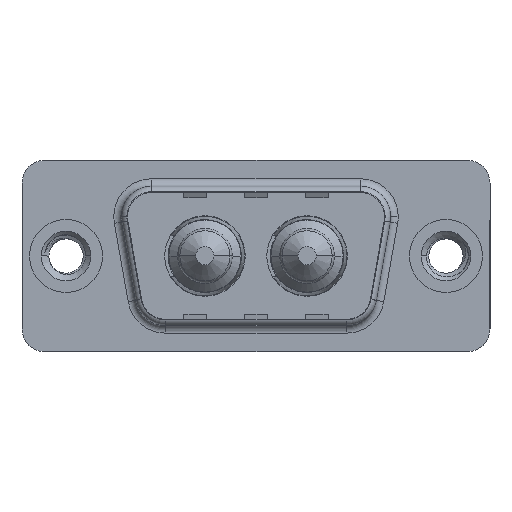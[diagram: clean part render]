
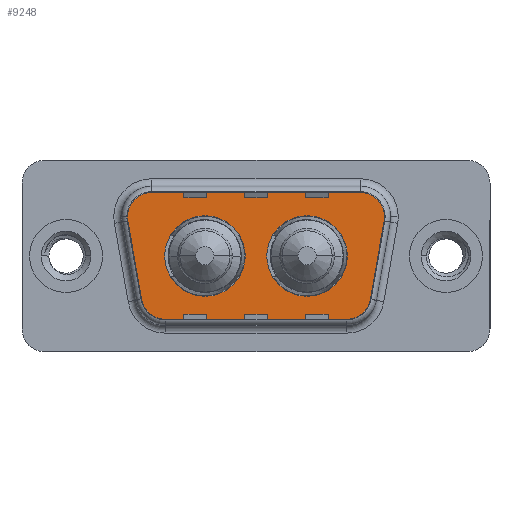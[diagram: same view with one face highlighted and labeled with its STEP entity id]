
A CAD part, top view. The second image highlights one B-rep face of the part: STEP entity #9248.
In plain terms, the highlighted planar face has unit normal (0, 0, 1).
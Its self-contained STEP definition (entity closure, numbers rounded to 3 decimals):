
#182 = CARTESIAN_POINT ( 'NONE',  ( 18.51, 0., 0. ) ) ;
#448 = DIRECTION ( 'NONE',  ( 1., 0., 0. ) ) ;
#459 = CARTESIAN_POINT ( 'NONE',  ( 3.466, 2.553, 0. ) ) ;
#536 = AXIS2_PLACEMENT_3D ( 'NONE', #2678, #3734, #14367 ) ;
#916 = VERTEX_POINT ( 'NONE', #13781 ) ;
#1003 = CARTESIAN_POINT ( 'NONE',  ( 4.489, -3.247, 0. ) ) ;
#1286 = LINE ( 'NONE', #11417, #12394 ) ;
#1322 = EDGE_CURVE ( 'NONE', #8747, #2855, #10840, .T. ) ;
#1399 = DIRECTION ( 'NONE',  ( 1., 0., 0. ) ) ;
#1548 = ORIENTED_EDGE ( 'NONE', *, *, #9249, .T. ) ;
#1556 = VERTEX_POINT ( 'NONE', #9598 ) ;
#1558 = CARTESIAN_POINT ( 'NONE',  ( 18.541, -4.9, 0. ) ) ;
#1772 = AXIS2_PLACEMENT_3D ( 'NONE', #13180, #13025, #5151 ) ;
#1902 = AXIS2_PLACEMENT_3D ( 'NONE', #4893, #12496, #5946 ) ;
#1916 = EDGE_CURVE ( 'NONE', #3289, #916, #9775, .T. ) ;
#2502 = AXIS2_PLACEMENT_3D ( 'NONE', #5964, #13618, #7005 ) ;
#2592 = ORIENTED_EDGE ( 'NONE', *, *, #5114, .T. ) ;
#2595 = CIRCLE ( 'NONE', #7024, 2. ) ;
#2678 = CARTESIAN_POINT ( 'NONE',  ( 19.564, 2.9, 0. ) ) ;
#2705 = AXIS2_PLACEMENT_3D ( 'NONE', #4806, #8030, #1399 ) ;
#2722 = DIRECTION ( 'NONE',  ( 0.174, -0.985, 0. ) ) ;
#2855 = VERTEX_POINT ( 'NONE', #13952 ) ;
#2955 = CARTESIAN_POINT ( 'NONE',  ( 21.534, 2.553, 0. ) ) ;
#3003 = ORIENTED_EDGE ( 'NONE', *, *, #4935, .T. ) ;
#3078 = VERTEX_POINT ( 'NONE', #5023 ) ;
#3113 = ORIENTED_EDGE ( 'NONE', *, *, #10744, .T. ) ;
#3155 = CARTESIAN_POINT ( 'NONE',  ( 5.436, 4.9, 0. ) ) ;
#3181 = DIRECTION ( 'NONE',  ( 1., 0., 0. ) ) ;
#3289 = VERTEX_POINT ( 'NONE', #182 ) ;
#3477 = ORIENTED_EDGE ( 'NONE', *, *, #8635, .F. ) ;
#3613 = AXIS2_PLACEMENT_3D ( 'NONE', #13808, #7171, #448 ) ;
#3653 = VERTEX_POINT ( 'NONE', #4293 ) ;
#3720 = CARTESIAN_POINT ( 'NONE',  ( 3.466, 2.553, 0. ) ) ;
#3734 = DIRECTION ( 'NONE',  ( 0., 0., 1. ) ) ;
#4022 = CARTESIAN_POINT ( 'NONE',  ( 20.511, -3.247, 0. ) ) ;
#4157 = CARTESIAN_POINT ( 'NONE',  ( 9.14, 0., 0. ) ) ;
#4293 = CARTESIAN_POINT ( 'NONE',  ( 19.564, 4.9, 0. ) ) ;
#4419 = FACE_OUTER_BOUND ( 'NONE', #11685, .T. ) ;
#4490 = AXIS2_PLACEMENT_3D ( 'NONE', #9485, #6674, #14259 ) ;
#4501 = CARTESIAN_POINT ( 'NONE',  ( 19.564, 2.9, 0. ) ) ;
#4584 = ORIENTED_EDGE ( 'NONE', *, *, #11109, .T. ) ;
#4750 = FACE_BOUND ( 'NONE', #14009, .T. ) ;
#4806 = CARTESIAN_POINT ( 'NONE',  ( 18.541, -2.9, 0. ) ) ;
#4855 = PLANE ( 'NONE',  #2705 ) ;
#4893 = CARTESIAN_POINT ( 'NONE',  ( 18.541, -2.9, 0. ) ) ;
#4935 = EDGE_CURVE ( 'NONE', #5301, #8747, #9007, .T. ) ;
#5023 = CARTESIAN_POINT ( 'NONE',  ( 11.79, 0., 0. ) ) ;
#5114 = EDGE_CURVE ( 'NONE', #6606, #8376, #10218, .T. ) ;
#5151 = DIRECTION ( 'NONE',  ( 1., 0., 0. ) ) ;
#5214 = DIRECTION ( 'NONE',  ( 0., 0., 1. ) ) ;
#5246 = DIRECTION ( 'NONE',  ( 1., 0., 0. ) ) ;
#5301 = VERTEX_POINT ( 'NONE', #4022 ) ;
#5488 = ORIENTED_EDGE ( 'NONE', *, *, #1322, .T. ) ;
#5946 = DIRECTION ( 'NONE',  ( 1., 0., 0. ) ) ;
#5964 = CARTESIAN_POINT ( 'NONE',  ( 9.14, 0., 0. ) ) ;
#6102 = ORIENTED_EDGE ( 'NONE', *, *, #6405, .T. ) ;
#6174 = EDGE_CURVE ( 'NONE', #8376, #1556, #8634, .T. ) ;
#6405 = EDGE_CURVE ( 'NONE', #2855, #3653, #2595, .T. ) ;
#6485 = CARTESIAN_POINT ( 'NONE',  ( 6.459, -4.9, 0. ) ) ;
#6562 = VERTEX_POINT ( 'NONE', #3155 ) ;
#6606 = VERTEX_POINT ( 'NONE', #459 ) ;
#6674 = DIRECTION ( 'NONE',  ( 0., 0., 1. ) ) ;
#6960 = CARTESIAN_POINT ( 'NONE',  ( 6.49, 0., 0. ) ) ;
#7005 = DIRECTION ( 'NONE',  ( 1., 0., 0. ) ) ;
#7024 = AXIS2_PLACEMENT_3D ( 'NONE', #4501, #14358, #13864 ) ;
#7074 = EDGE_LOOP ( 'NONE', ( #8391, #11410 ) ) ;
#7171 = DIRECTION ( 'NONE',  ( 0., 0., 1. ) ) ;
#7727 = ORIENTED_EDGE ( 'NONE', *, *, #12026, .F. ) ;
#8030 = DIRECTION ( 'NONE',  ( 0., 0., 1. ) ) ;
#8376 = VERTEX_POINT ( 'NONE', #1003 ) ;
#8391 = ORIENTED_EDGE ( 'NONE', *, *, #1916, .F. ) ;
#8438 = ORIENTED_EDGE ( 'NONE', *, *, #9271, .T. ) ;
#8634 = CIRCLE ( 'NONE', #4490, 2. ) ;
#8635 = EDGE_CURVE ( 'NONE', #10497, #3078, #12411, .T. ) ;
#8661 = VECTOR ( 'NONE', #9678, 1000. ) ;
#8747 = VERTEX_POINT ( 'NONE', #13722 ) ;
#8895 = AXIS2_PLACEMENT_3D ( 'NONE', #4157, #11777, #5246 ) ;
#9007 = LINE ( 'NONE', #2955, #8661 ) ;
#9226 = DIRECTION ( 'NONE',  ( -1., 0., 0. ) ) ;
#9248 = ADVANCED_FACE ( 'NONE', ( #10145, #4750, #4419 ), #4855, .T. ) ;
#9249 = EDGE_CURVE ( 'NONE', #11093, #5301, #9809, .T. ) ;
#9271 = EDGE_CURVE ( 'NONE', #3653, #6562, #1286, .T. ) ;
#9485 = CARTESIAN_POINT ( 'NONE',  ( 6.459, -2.9, 0. ) ) ;
#9504 = EDGE_CURVE ( 'NONE', #916, #3289, #11034, .T. ) ;
#9598 = CARTESIAN_POINT ( 'NONE',  ( 6.459, -4.9, 0. ) ) ;
#9678 = DIRECTION ( 'NONE',  ( 0.174, 0.985, 0. ) ) ;
#9775 = CIRCLE ( 'NONE', #1772, 2.65 ) ;
#9809 = CIRCLE ( 'NONE', #1902, 2. ) ;
#9962 = VECTOR ( 'NONE', #3181, 1000. ) ;
#10145 = FACE_BOUND ( 'NONE', #7074, .T. ) ;
#10218 = LINE ( 'NONE', #3720, #13482 ) ;
#10320 = LINE ( 'NONE', #6485, #9962 ) ;
#10497 = VERTEX_POINT ( 'NONE', #6960 ) ;
#10744 = EDGE_CURVE ( 'NONE', #1556, #11093, #10320, .T. ) ;
#10840 = CIRCLE ( 'NONE', #536, 2. ) ;
#11034 = CIRCLE ( 'NONE', #13023, 2.65 ) ;
#11093 = VERTEX_POINT ( 'NONE', #1558 ) ;
#11109 = EDGE_CURVE ( 'NONE', #6562, #6606, #13050, .T. ) ;
#11410 = ORIENTED_EDGE ( 'NONE', *, *, #9504, .F. ) ;
#11417 = CARTESIAN_POINT ( 'NONE',  ( 5.436, 4.9, 0. ) ) ;
#11685 = EDGE_LOOP ( 'NONE', ( #1548, #3003, #5488, #6102, #8438, #4584, #2592, #13427, #3113 ) ) ;
#11742 = CARTESIAN_POINT ( 'NONE',  ( 15.86, 0., 0. ) ) ;
#11777 = DIRECTION ( 'NONE',  ( 0., 0., 1. ) ) ;
#12026 = EDGE_CURVE ( 'NONE', #3078, #10497, #13035, .T. ) ;
#12394 = VECTOR ( 'NONE', #9226, 1000. ) ;
#12411 = CIRCLE ( 'NONE', #2502, 2.65 ) ;
#12496 = DIRECTION ( 'NONE',  ( 0., 0., 1. ) ) ;
#12813 = DIRECTION ( 'NONE',  ( 1., 0., 0. ) ) ;
#13023 = AXIS2_PLACEMENT_3D ( 'NONE', #11742, #5214, #12813 ) ;
#13025 = DIRECTION ( 'NONE',  ( 0., 0., 1. ) ) ;
#13035 = CIRCLE ( 'NONE', #8895, 2.65 ) ;
#13050 = CIRCLE ( 'NONE', #3613, 2. ) ;
#13180 = CARTESIAN_POINT ( 'NONE',  ( 15.86, 0., 0. ) ) ;
#13427 = ORIENTED_EDGE ( 'NONE', *, *, #6174, .T. ) ;
#13482 = VECTOR ( 'NONE', #2722, 1000. ) ;
#13618 = DIRECTION ( 'NONE',  ( 0., 0., 1. ) ) ;
#13722 = CARTESIAN_POINT ( 'NONE',  ( 21.534, 2.553, 0. ) ) ;
#13781 = CARTESIAN_POINT ( 'NONE',  ( 13.21, 0., 0. ) ) ;
#13808 = CARTESIAN_POINT ( 'NONE',  ( 5.436, 2.9, 0. ) ) ;
#13864 = DIRECTION ( 'NONE',  ( -1., 0., 0. ) ) ;
#13952 = CARTESIAN_POINT ( 'NONE',  ( 21.564, 2.9, 0. ) ) ;
#14009 = EDGE_LOOP ( 'NONE', ( #7727, #3477 ) ) ;
#14259 = DIRECTION ( 'NONE',  ( -1., 0., 0. ) ) ;
#14358 = DIRECTION ( 'NONE',  ( 0., 0., 1. ) ) ;
#14367 = DIRECTION ( 'NONE',  ( -1., 0., 0. ) ) ;
